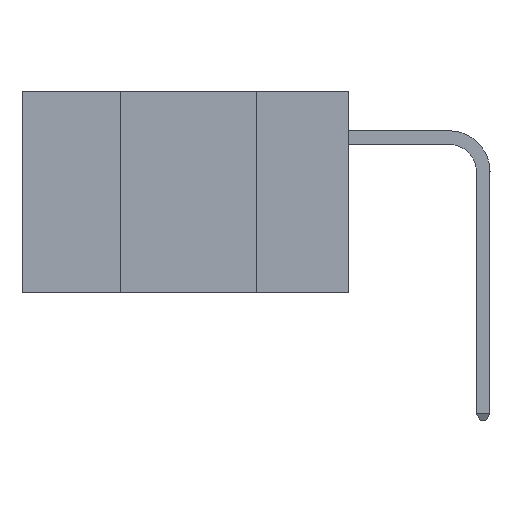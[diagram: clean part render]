
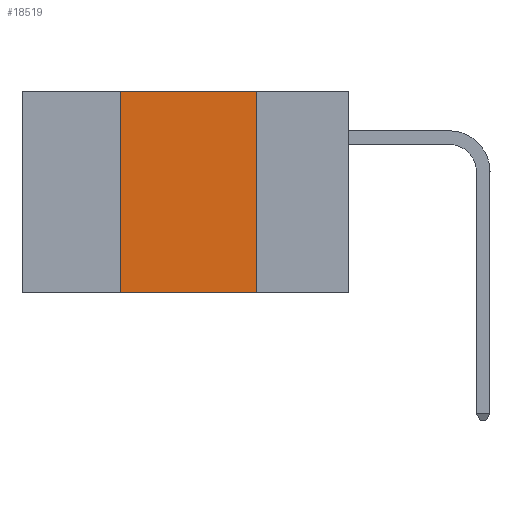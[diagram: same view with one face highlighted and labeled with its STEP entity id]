
A CAD part, left-side view. The second image highlights one B-rep face of the part: STEP entity #18519.
In plain terms, the highlighted planar face has unit normal (-1, 0, 0).
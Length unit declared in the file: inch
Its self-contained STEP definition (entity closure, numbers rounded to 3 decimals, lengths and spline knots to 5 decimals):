
#135 = CARTESIAN_POINT ( 'NONE',  ( 0., 0.17, 0. ) ) ;
#166 = LINE ( 'NONE', #812, #28828 ) ;
#584 = EDGE_LOOP ( 'NONE', ( #21714, #1027, #30495, #20480 ) ) ;
#812 = CARTESIAN_POINT ( 'NONE',  ( 0., 0.6, -0.37 ) ) ;
#1027 = ORIENTED_EDGE ( 'NONE', *, *, #4111, .F. ) ;
#2258 = DIRECTION ( 'NONE',  ( 0., 0., 1. ) ) ;
#4111 = EDGE_CURVE ( 'NONE', #31872, #8359, #19067, .T. ) ;
#4406 = DIRECTION ( 'NONE',  ( 0., -1., 0. ) ) ;
#8175 = DIRECTION ( 'NONE',  ( 1., 0., 0. ) ) ;
#8359 = VERTEX_POINT ( 'NONE', #135 ) ;
#8851 = CARTESIAN_POINT ( 'NONE',  ( 0., 0.42, 0. ) ) ;
#9477 = VECTOR ( 'NONE', #2258, 39.37008 ) ;
#11485 = DIRECTION ( 'NONE',  ( 0., 0., -1. ) ) ;
#13762 = CARTESIAN_POINT ( 'NONE',  ( 0., 0.17, -0.37 ) ) ;
#14324 = DIRECTION ( 'NONE',  ( 0., -1., 0. ) ) ;
#15051 = CARTESIAN_POINT ( 'NONE',  ( 0., 0.42, -0.37 ) ) ;
#16165 = PLANE ( 'NONE',  #28002 ) ;
#18519 = ADVANCED_FACE ( 'NONE', ( #32722 ), #16165, .F. ) ;
#18742 = LINE ( 'NONE', #27510, #25011 ) ;
#19067 = LINE ( 'NONE', #20555, #19938 ) ;
#19938 = VECTOR ( 'NONE', #4406, 39.37008 ) ;
#20480 = ORIENTED_EDGE ( 'NONE', *, *, #29331, .T. ) ;
#20555 = CARTESIAN_POINT ( 'NONE',  ( 0., 0.6, 0. ) ) ;
#20907 = EDGE_CURVE ( 'NONE', #8359, #25572, #18742, .T. ) ;
#21126 = CARTESIAN_POINT ( 'NONE',  ( 0., 0.42, 0. ) ) ;
#21714 = ORIENTED_EDGE ( 'NONE', *, *, #20907, .F. ) ;
#24230 = CARTESIAN_POINT ( 'NONE',  ( 0., 0.6, 0. ) ) ;
#24569 = LINE ( 'NONE', #21126, #9477 ) ;
#25011 = VECTOR ( 'NONE', #11485, 39.37008 ) ;
#25572 = VERTEX_POINT ( 'NONE', #13762 ) ;
#26908 = DIRECTION ( 'NONE',  ( 0., 0., -1. ) ) ;
#27510 = CARTESIAN_POINT ( 'NONE',  ( 0., 0.17, 0. ) ) ;
#28002 = AXIS2_PLACEMENT_3D ( 'NONE', #24230, #8175, #26908 ) ;
#28828 = VECTOR ( 'NONE', #14324, 39.37008 ) ;
#29331 = EDGE_CURVE ( 'NONE', #32045, #25572, #166, .T. ) ;
#30495 = ORIENTED_EDGE ( 'NONE', *, *, #30917, .F. ) ;
#30917 = EDGE_CURVE ( 'NONE', #32045, #31872, #24569, .T. ) ;
#31872 = VERTEX_POINT ( 'NONE', #8851 ) ;
#32045 = VERTEX_POINT ( 'NONE', #15051 ) ;
#32722 = FACE_OUTER_BOUND ( 'NONE', #584, .T. ) ;
